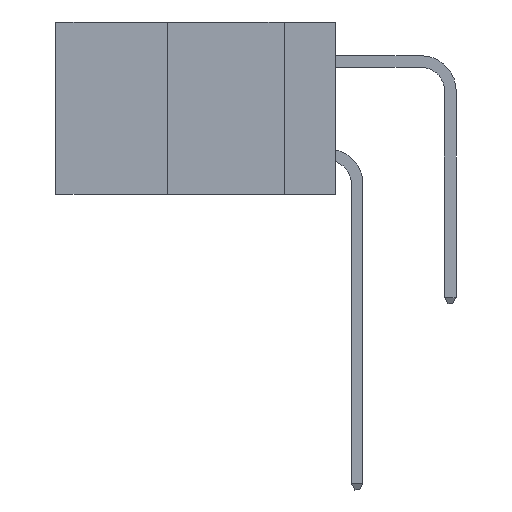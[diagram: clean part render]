
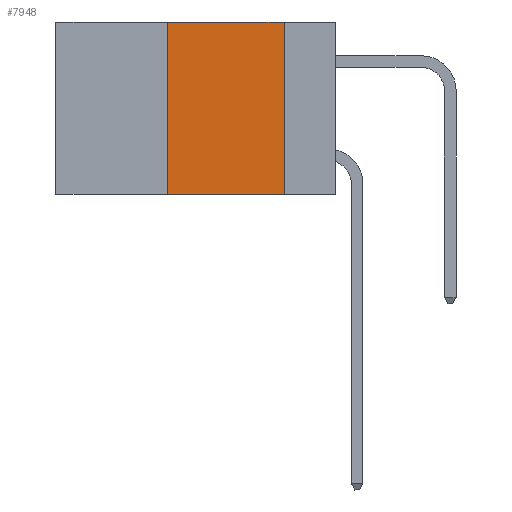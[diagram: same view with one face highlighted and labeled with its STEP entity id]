
A CAD part, left-side view. The second image highlights one B-rep face of the part: STEP entity #7948.
In plain terms, the highlighted planar face has unit normal (-1, 0, 0).
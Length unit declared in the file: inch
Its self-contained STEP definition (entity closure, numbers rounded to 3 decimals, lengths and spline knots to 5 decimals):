
#380 = DIRECTION ( 'NONE',  ( 0., -1., 0. ) ) ;
#440 = ORIENTED_EDGE ( 'NONE', *, *, #11879, .F. ) ;
#677 = VECTOR ( 'NONE', #5854, 39.37008 ) ;
#821 = ORIENTED_EDGE ( 'NONE', *, *, #10784, .T. ) ;
#1368 = CARTESIAN_POINT ( 'NONE',  ( 0., 0.36, 0. ) ) ;
#1676 = CARTESIAN_POINT ( 'NONE',  ( 0., 0.11, 0. ) ) ;
#2423 = ORIENTED_EDGE ( 'NONE', *, *, #13183, .F. ) ;
#2785 = VECTOR ( 'NONE', #380, 39.37008 ) ;
#3074 = VERTEX_POINT ( 'NONE', #3421 ) ;
#3188 = PLANE ( 'NONE',  #10246 ) ;
#3401 = VERTEX_POINT ( 'NONE', #11731 ) ;
#3421 = CARTESIAN_POINT ( 'NONE',  ( 0., 0.36, -0.37 ) ) ;
#3604 = LINE ( 'NONE', #4166, #9455 ) ;
#4166 = CARTESIAN_POINT ( 'NONE',  ( 0., 0.6, 0. ) ) ;
#4316 = DIRECTION ( 'NONE',  ( 0., 0., -1. ) ) ;
#4932 = CARTESIAN_POINT ( 'NONE',  ( 0., 0.6, -0.37 ) ) ;
#5854 = DIRECTION ( 'NONE',  ( 0., 0., 1. ) ) ;
#6336 = EDGE_CURVE ( 'NONE', #12711, #12888, #6870, .T. ) ;
#6502 = CARTESIAN_POINT ( 'NONE',  ( 0., 0.6, 0. ) ) ;
#6870 = LINE ( 'NONE', #11623, #9402 ) ;
#7745 = EDGE_LOOP ( 'NONE', ( #8423, #2423, #440, #821 ) ) ;
#7948 = ADVANCED_FACE ( 'NONE', ( #9858 ), #3188, .F. ) ;
#8280 = LINE ( 'NONE', #4932, #2785 ) ;
#8423 = ORIENTED_EDGE ( 'NONE', *, *, #6336, .F. ) ;
#9402 = VECTOR ( 'NONE', #13007, 39.37008 ) ;
#9455 = VECTOR ( 'NONE', #11656, 39.37008 ) ;
#9858 = FACE_OUTER_BOUND ( 'NONE', #7745, .T. ) ;
#10246 = AXIS2_PLACEMENT_3D ( 'NONE', #6502, #10788, #4316 ) ;
#10784 = EDGE_CURVE ( 'NONE', #3074, #12888, #8280, .T. ) ;
#10788 = DIRECTION ( 'NONE',  ( 1., 0., 0. ) ) ;
#11623 = CARTESIAN_POINT ( 'NONE',  ( 0., 0.11, 0. ) ) ;
#11656 = DIRECTION ( 'NONE',  ( 0., -1., 0. ) ) ;
#11731 = CARTESIAN_POINT ( 'NONE',  ( 0., 0.36, 0. ) ) ;
#11879 = EDGE_CURVE ( 'NONE', #3074, #3401, #12843, .T. ) ;
#11948 = CARTESIAN_POINT ( 'NONE',  ( 0., 0.11, -0.37 ) ) ;
#12711 = VERTEX_POINT ( 'NONE', #1676 ) ;
#12843 = LINE ( 'NONE', #1368, #677 ) ;
#12888 = VERTEX_POINT ( 'NONE', #11948 ) ;
#13007 = DIRECTION ( 'NONE',  ( 0., 0., -1. ) ) ;
#13183 = EDGE_CURVE ( 'NONE', #3401, #12711, #3604, .T. ) ;
